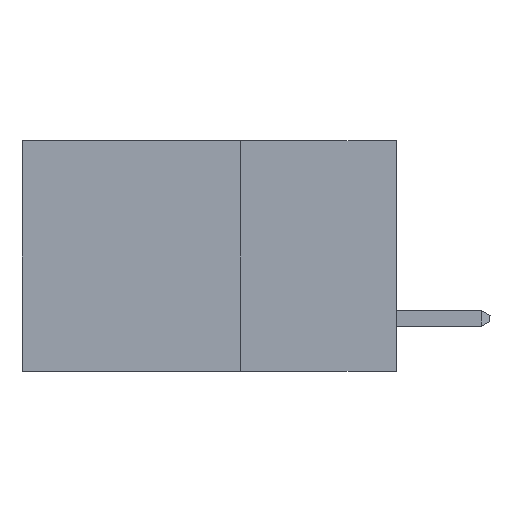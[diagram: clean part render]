
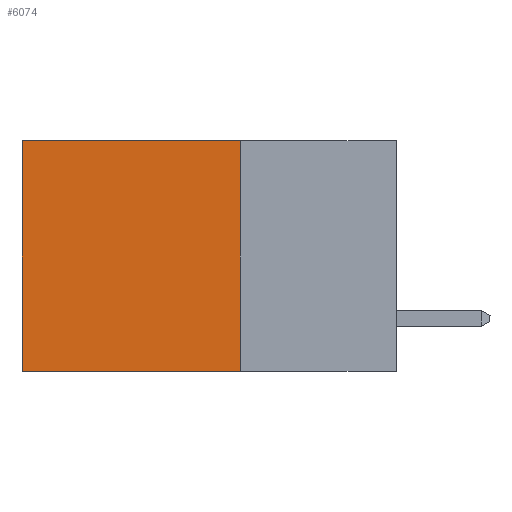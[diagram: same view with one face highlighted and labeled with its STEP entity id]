
A CAD part, left-side view. The second image highlights one B-rep face of the part: STEP entity #6074.
In plain terms, the highlighted planar face has unit normal (-1, 0, 0).
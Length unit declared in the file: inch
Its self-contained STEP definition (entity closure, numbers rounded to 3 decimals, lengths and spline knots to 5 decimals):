
#1018 = AXIS2_PLACEMENT_3D ( 'NONE', #7381, #7264, #7493 ) ;
#1108 = ORIENTED_EDGE ( 'NONE', *, *, #15409, .F. ) ;
#1206 = VECTOR ( 'NONE', #12586, 39.37008 ) ;
#2083 = FACE_OUTER_BOUND ( 'NONE', #14356, .T. ) ;
#3504 = CARTESIAN_POINT ( 'NONE',  ( 0.2615, 0.25, -0.37 ) ) ;
#3846 = LINE ( 'NONE', #3504, #18686 ) ;
#4081 = DIRECTION ( 'NONE',  ( 0., 0., -1. ) ) ;
#4188 = CARTESIAN_POINT ( 'NONE',  ( 0.2615, 0.25, -0.37 ) ) ;
#4254 = PLANE ( 'NONE',  #1018 ) ;
#5350 = VECTOR ( 'NONE', #4081, 39.37008 ) ;
#6074 = ADVANCED_FACE ( 'NONE', ( #2083 ), #4254, .F. ) ;
#7264 = DIRECTION ( 'NONE',  ( 1., 0., 0. ) ) ;
#7381 = CARTESIAN_POINT ( 'NONE',  ( 0.2615, 0.25, -0.37 ) ) ;
#7493 = DIRECTION ( 'NONE',  ( 0., 0., -1. ) ) ;
#8963 = VECTOR ( 'NONE', #21238, 39.37008 ) ;
#9107 = LINE ( 'NONE', #16172, #8963 ) ;
#9798 = ORIENTED_EDGE ( 'NONE', *, *, #10142, .T. ) ;
#10142 = EDGE_CURVE ( 'NONE', #18119, #14791, #17562, .T. ) ;
#10373 = CARTESIAN_POINT ( 'NONE',  ( 0.2615, 0.6, -0.37 ) ) ;
#10382 = VERTEX_POINT ( 'NONE', #21956 ) ;
#10686 = EDGE_CURVE ( 'NONE', #11284, #18119, #9107, .T. ) ;
#11284 = VERTEX_POINT ( 'NONE', #20050 ) ;
#12121 = ORIENTED_EDGE ( 'NONE', *, *, #16940, .F. ) ;
#12586 = DIRECTION ( 'NONE',  ( 0., 0., -1. ) ) ;
#14356 = EDGE_LOOP ( 'NONE', ( #9798, #12121, #1108, #15892 ) ) ;
#14791 = VERTEX_POINT ( 'NONE', #10373 ) ;
#15409 = EDGE_CURVE ( 'NONE', #11284, #10382, #20028, .T. ) ;
#15892 = ORIENTED_EDGE ( 'NONE', *, *, #10686, .T. ) ;
#16172 = CARTESIAN_POINT ( 'NONE',  ( 0.2615, 0.25, 0. ) ) ;
#16940 = EDGE_CURVE ( 'NONE', #10382, #14791, #3846, .T. ) ;
#17478 = DIRECTION ( 'NONE',  ( 0., 1., 0. ) ) ;
#17562 = LINE ( 'NONE', #17682, #1206 ) ;
#17682 = CARTESIAN_POINT ( 'NONE',  ( 0.2615, 0.6, -0.37 ) ) ;
#18119 = VERTEX_POINT ( 'NONE', #18623 ) ;
#18623 = CARTESIAN_POINT ( 'NONE',  ( 0.2615, 0.6, 0. ) ) ;
#18686 = VECTOR ( 'NONE', #17478, 39.37008 ) ;
#20028 = LINE ( 'NONE', #4188, #5350 ) ;
#20050 = CARTESIAN_POINT ( 'NONE',  ( 0.2615, 0.25, 0. ) ) ;
#21238 = DIRECTION ( 'NONE',  ( 0., 1., 0. ) ) ;
#21956 = CARTESIAN_POINT ( 'NONE',  ( 0.2615, 0.25, -0.37 ) ) ;
